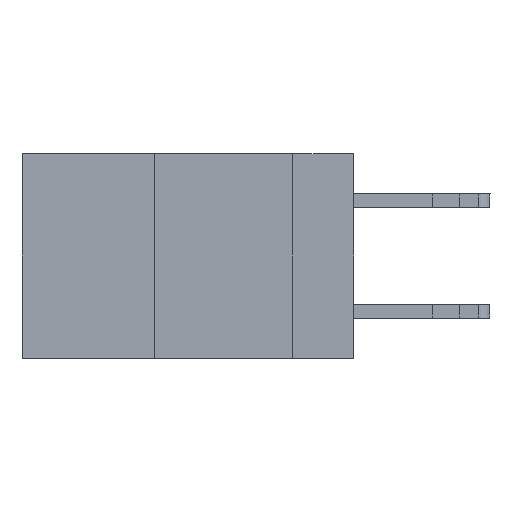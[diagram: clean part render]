
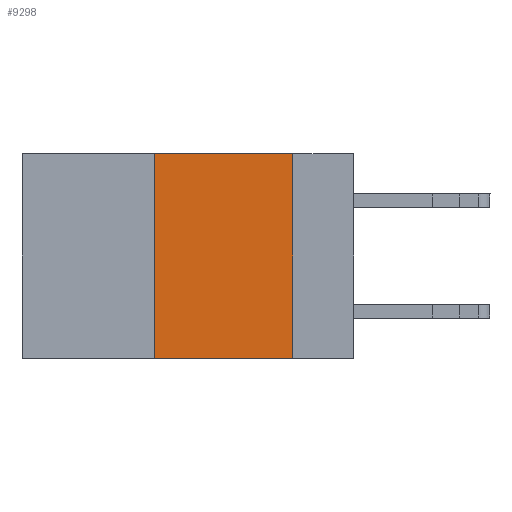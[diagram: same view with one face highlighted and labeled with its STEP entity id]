
A CAD part, left-side view. The second image highlights one B-rep face of the part: STEP entity #9298.
In plain terms, the highlighted planar face has unit normal (-1, 0, 0).
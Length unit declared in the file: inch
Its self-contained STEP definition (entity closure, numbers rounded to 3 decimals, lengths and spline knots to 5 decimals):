
#1431 = VECTOR ( 'NONE', #6490, 39.37008 ) ;
#2407 = DIRECTION ( 'NONE',  ( 0., 0., -1. ) ) ;
#2730 = VERTEX_POINT ( 'NONE', #16202 ) ;
#2997 = ORIENTED_EDGE ( 'NONE', *, *, #13888, .F. ) ;
#4243 = EDGE_CURVE ( 'NONE', #26869, #2730, #11938, .T. ) ;
#5341 = ORIENTED_EDGE ( 'NONE', *, *, #19220, .F. ) ;
#6490 = DIRECTION ( 'NONE',  ( 0., -1., 0. ) ) ;
#7395 = CARTESIAN_POINT ( 'NONE',  ( 0., 0.36, 0. ) ) ;
#7808 = ORIENTED_EDGE ( 'NONE', *, *, #11539, .T. ) ;
#8795 = CARTESIAN_POINT ( 'NONE',  ( 0., 0.11, 0. ) ) ;
#9298 = ADVANCED_FACE ( 'NONE', ( #23331 ), #21316, .F. ) ;
#9481 = VECTOR ( 'NONE', #24633, 39.37008 ) ;
#10709 = LINE ( 'NONE', #8795, #20866 ) ;
#11165 = AXIS2_PLACEMENT_3D ( 'NONE', #23192, #14894, #23597 ) ;
#11242 = VECTOR ( 'NONE', #21493, 39.37008 ) ;
#11539 = EDGE_CURVE ( 'NONE', #14634, #24644, #14695, .T. ) ;
#11854 = CARTESIAN_POINT ( 'NONE',  ( 0., 0.36, -0.37 ) ) ;
#11938 = LINE ( 'NONE', #24763, #9481 ) ;
#13249 = CARTESIAN_POINT ( 'NONE',  ( 0., 0.11, -0.37 ) ) ;
#13841 = EDGE_LOOP ( 'NONE', ( #2997, #19284, #5341, #7808 ) ) ;
#13888 = EDGE_CURVE ( 'NONE', #2730, #24644, #10709, .T. ) ;
#14634 = VERTEX_POINT ( 'NONE', #11854 ) ;
#14695 = LINE ( 'NONE', #25200, #1431 ) ;
#14894 = DIRECTION ( 'NONE',  ( 1., 0., 0. ) ) ;
#16202 = CARTESIAN_POINT ( 'NONE',  ( 0., 0.11, 0. ) ) ;
#19220 = EDGE_CURVE ( 'NONE', #14634, #26869, #23932, .T. ) ;
#19284 = ORIENTED_EDGE ( 'NONE', *, *, #4243, .F. ) ;
#20866 = VECTOR ( 'NONE', #2407, 39.37008 ) ;
#21316 = PLANE ( 'NONE',  #11165 ) ;
#21493 = DIRECTION ( 'NONE',  ( 0., 0., 1. ) ) ;
#21911 = CARTESIAN_POINT ( 'NONE',  ( 0., 0.36, 0. ) ) ;
#23192 = CARTESIAN_POINT ( 'NONE',  ( 0., 0.6, 0. ) ) ;
#23331 = FACE_OUTER_BOUND ( 'NONE', #13841, .T. ) ;
#23597 = DIRECTION ( 'NONE',  ( 0., 0., -1. ) ) ;
#23932 = LINE ( 'NONE', #21911, #11242 ) ;
#24633 = DIRECTION ( 'NONE',  ( 0., -1., 0. ) ) ;
#24644 = VERTEX_POINT ( 'NONE', #13249 ) ;
#24763 = CARTESIAN_POINT ( 'NONE',  ( 0., 0.6, 0. ) ) ;
#25200 = CARTESIAN_POINT ( 'NONE',  ( 0., 0.6, -0.37 ) ) ;
#26869 = VERTEX_POINT ( 'NONE', #7395 ) ;
